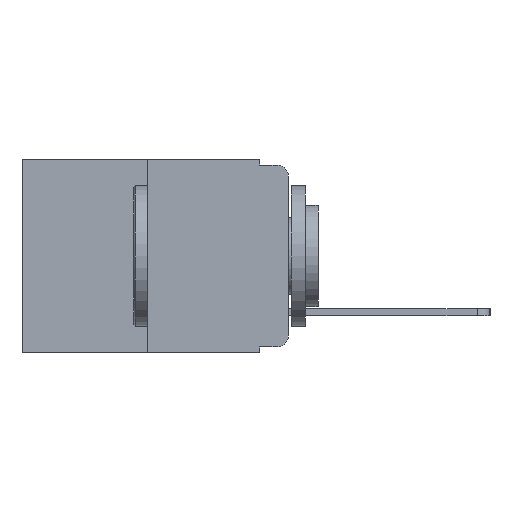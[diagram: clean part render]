
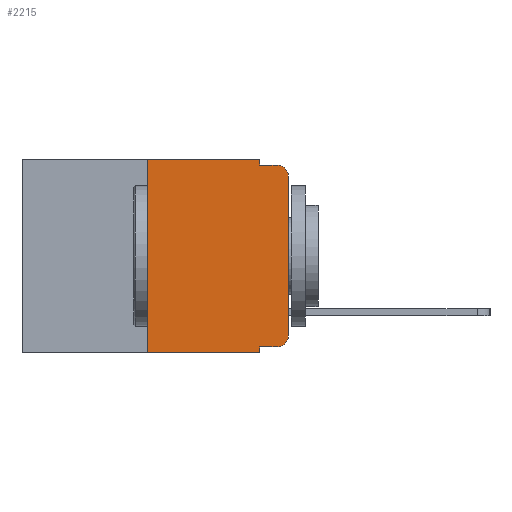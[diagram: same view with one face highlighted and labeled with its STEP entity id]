
A CAD part, left-side view. The second image highlights one B-rep face of the part: STEP entity #2215.
In plain terms, the highlighted planar face has unit normal (-1, 0, 0).
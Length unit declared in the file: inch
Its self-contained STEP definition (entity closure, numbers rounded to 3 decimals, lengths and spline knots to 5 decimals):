
#34 = CIRCLE ( 'NONE', #5438, 0.02 ) ;
#67 = DIRECTION ( 'NONE',  ( 0., 0., -1. ) ) ;
#634 = ORIENTED_EDGE ( 'NONE', *, *, #14033, .F. ) ;
#883 = EDGE_CURVE ( 'NONE', #1684, #4081, #5629, .T. ) ;
#1476 = CARTESIAN_POINT ( 'NONE',  ( 0., 0.051, -0.343 ) ) ;
#1682 = CARTESIAN_POINT ( 'NONE',  ( 0., 0., -0.313 ) ) ;
#1684 = VERTEX_POINT ( 'NONE', #8333 ) ;
#1850 = EDGE_CURVE ( 'NONE', #2353, #4081, #8822, .T. ) ;
#1915 = CARTESIAN_POINT ( 'NONE',  ( 0., 0., 0. ) ) ;
#1984 = DIRECTION ( 'NONE',  ( 0., 0., -1. ) ) ;
#2073 = AXIS2_PLACEMENT_3D ( 'NONE', #12055, #6721, #67 ) ;
#2215 = ADVANCED_FACE ( 'NONE', ( #13840 ), #13780, .F. ) ;
#2353 = VERTEX_POINT ( 'NONE', #4585 ) ;
#2724 = VECTOR ( 'NONE', #4982, 39.37008 ) ;
#2763 = EDGE_CURVE ( 'NONE', #4555, #2353, #11212, .T. ) ;
#2838 = ORIENTED_EDGE ( 'NONE', *, *, #1850, .T. ) ;
#3134 = VERTEX_POINT ( 'NONE', #1476 ) ;
#3234 = DIRECTION ( 'NONE',  ( 0., 0., 1. ) ) ;
#3673 = VERTEX_POINT ( 'NONE', #7927 ) ;
#3797 = CARTESIAN_POINT ( 'NONE',  ( 0., 0.051, -0.333 ) ) ;
#3893 = DIRECTION ( 'NONE',  ( 0., -1., 0. ) ) ;
#3983 = VERTEX_POINT ( 'NONE', #3797 ) ;
#4081 = VERTEX_POINT ( 'NONE', #7202 ) ;
#4103 = EDGE_CURVE ( 'NONE', #7413, #3134, #5882, .T. ) ;
#4207 = VERTEX_POINT ( 'NONE', #10639 ) ;
#4225 = CARTESIAN_POINT ( 'NONE',  ( 0., 0.25, 0. ) ) ;
#4555 = VERTEX_POINT ( 'NONE', #1682 ) ;
#4569 = ORIENTED_EDGE ( 'NONE', *, *, #14106, .F. ) ;
#4585 = CARTESIAN_POINT ( 'NONE',  ( 0., 0., -0.03 ) ) ;
#4939 = CARTESIAN_POINT ( 'NONE',  ( 0., 0.473, 0. ) ) ;
#4982 = DIRECTION ( 'NONE',  ( 0., -1., 0. ) ) ;
#5007 = AXIS2_PLACEMENT_3D ( 'NONE', #6242, #7305, #14786 ) ;
#5183 = VECTOR ( 'NONE', #9430, 39.37008 ) ;
#5438 = AXIS2_PLACEMENT_3D ( 'NONE', #6334, #13874, #7396 ) ;
#5462 = ORIENTED_EDGE ( 'NONE', *, *, #13441, .F. ) ;
#5540 = LINE ( 'NONE', #6825, #13503 ) ;
#5629 = LINE ( 'NONE', #6949, #13589 ) ;
#5882 = LINE ( 'NONE', #10592, #13500 ) ;
#6140 = ORIENTED_EDGE ( 'NONE', *, *, #12752, .T. ) ;
#6242 = CARTESIAN_POINT ( 'NONE',  ( 0., 0.473, 0. ) ) ;
#6334 = CARTESIAN_POINT ( 'NONE',  ( 0., 0.02, -0.313 ) ) ;
#6379 = VECTOR ( 'NONE', #1984, 39.37008 ) ;
#6529 = CARTESIAN_POINT ( 'NONE',  ( 0., 0.051, 0. ) ) ;
#6721 = DIRECTION ( 'NONE',  ( -1., 0., 0. ) ) ;
#6825 = CARTESIAN_POINT ( 'NONE',  ( 0., 0.051, -0.333 ) ) ;
#6949 = CARTESIAN_POINT ( 'NONE',  ( 0., 0.051, -0.01 ) ) ;
#7144 = ORIENTED_EDGE ( 'NONE', *, *, #12043, .T. ) ;
#7179 = VECTOR ( 'NONE', #8714, 39.37008 ) ;
#7202 = CARTESIAN_POINT ( 'NONE',  ( 0., 0.02, -0.01 ) ) ;
#7305 = DIRECTION ( 'NONE',  ( 1., 0., 0. ) ) ;
#7396 = DIRECTION ( 'NONE',  ( 0., 0., -1. ) ) ;
#7413 = VERTEX_POINT ( 'NONE', #8366 ) ;
#7754 = DIRECTION ( 'NONE',  ( 0., -1., 0. ) ) ;
#7896 = VERTEX_POINT ( 'NONE', #4225 ) ;
#7908 = DIRECTION ( 'NONE',  ( 0., -1., 0. ) ) ;
#7927 = CARTESIAN_POINT ( 'NONE',  ( 0., 0.02, -0.333 ) ) ;
#7990 = ORIENTED_EDGE ( 'NONE', *, *, #4103, .T. ) ;
#8333 = CARTESIAN_POINT ( 'NONE',  ( 0., 0.051, -0.01 ) ) ;
#8366 = CARTESIAN_POINT ( 'NONE',  ( 0., 0.25, -0.343 ) ) ;
#8394 = LINE ( 'NONE', #13668, #5183 ) ;
#8714 = DIRECTION ( 'NONE',  ( 0., 0., -1. ) ) ;
#8822 = CIRCLE ( 'NONE', #2073, 0.02 ) ;
#9297 = LINE ( 'NONE', #13183, #6379 ) ;
#9430 = DIRECTION ( 'NONE',  ( 0., 0., 1. ) ) ;
#10169 = LINE ( 'NONE', #6529, #7179 ) ;
#10287 = ORIENTED_EDGE ( 'NONE', *, *, #883, .F. ) ;
#10592 = CARTESIAN_POINT ( 'NONE',  ( 0., 0.473, -0.343 ) ) ;
#10639 = CARTESIAN_POINT ( 'NONE',  ( 0., 0.051, 0. ) ) ;
#11212 = LINE ( 'NONE', #1915, #13659 ) ;
#11617 = ORIENTED_EDGE ( 'NONE', *, *, #14776, .F. ) ;
#12016 = LINE ( 'NONE', #4939, #2724 ) ;
#12043 = EDGE_CURVE ( 'NONE', #3673, #4555, #34, .T. ) ;
#12055 = CARTESIAN_POINT ( 'NONE',  ( 0., 0.02, -0.03 ) ) ;
#12338 = EDGE_LOOP ( 'NONE', ( #13884, #2838, #10287, #11617, #634, #4569, #7990, #5462, #6140, #7144 ) ) ;
#12752 = EDGE_CURVE ( 'NONE', #3983, #3673, #5540, .T. ) ;
#13183 = CARTESIAN_POINT ( 'NONE',  ( 0., 0.051, 0. ) ) ;
#13441 = EDGE_CURVE ( 'NONE', #3983, #3134, #9297, .T. ) ;
#13500 = VECTOR ( 'NONE', #3893, 39.37008 ) ;
#13503 = VECTOR ( 'NONE', #7908, 39.37008 ) ;
#13589 = VECTOR ( 'NONE', #7754, 39.37008 ) ;
#13659 = VECTOR ( 'NONE', #3234, 39.37008 ) ;
#13668 = CARTESIAN_POINT ( 'NONE',  ( 0., 0.25, 0. ) ) ;
#13780 = PLANE ( 'NONE',  #5007 ) ;
#13840 = FACE_OUTER_BOUND ( 'NONE', #12338, .T. ) ;
#13874 = DIRECTION ( 'NONE',  ( -1., 0., 0. ) ) ;
#13884 = ORIENTED_EDGE ( 'NONE', *, *, #2763, .T. ) ;
#14033 = EDGE_CURVE ( 'NONE', #7896, #4207, #12016, .T. ) ;
#14106 = EDGE_CURVE ( 'NONE', #7413, #7896, #8394, .T. ) ;
#14776 = EDGE_CURVE ( 'NONE', #4207, #1684, #10169, .T. ) ;
#14786 = DIRECTION ( 'NONE',  ( 0., 0., -1. ) ) ;
